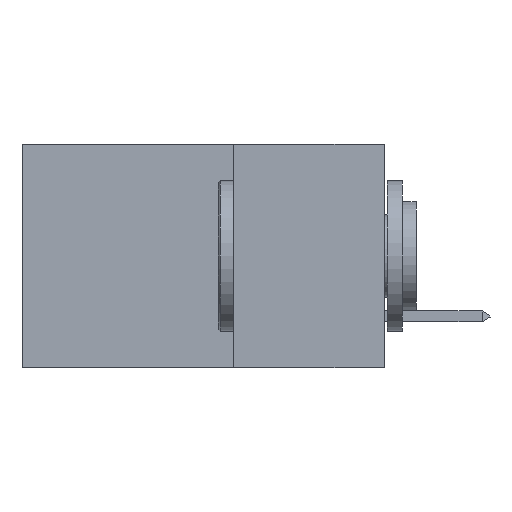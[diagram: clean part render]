
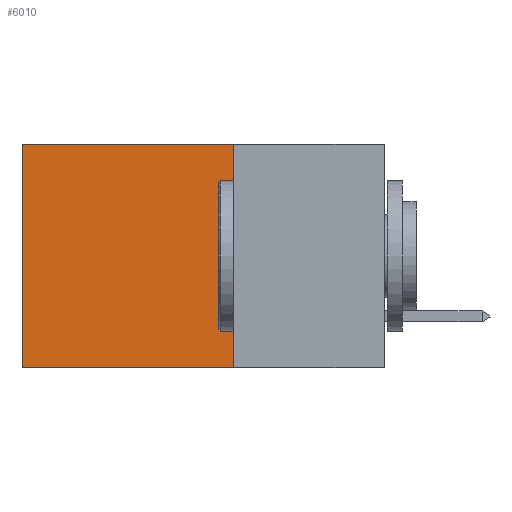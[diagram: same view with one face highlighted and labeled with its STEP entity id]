
A CAD part, left-side view. The second image highlights one B-rep face of the part: STEP entity #6010.
In plain terms, the highlighted planar face has unit normal (-1, 0, 0).
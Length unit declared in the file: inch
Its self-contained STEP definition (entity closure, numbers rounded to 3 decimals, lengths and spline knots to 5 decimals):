
#478 = EDGE_CURVE ( 'NONE', #10858, #31970, #16293, .T. ) ;
#938 = FACE_OUTER_BOUND ( 'NONE', #32908, .T. ) ;
#1613 = ORIENTED_EDGE ( 'NONE', *, *, #37143, .F. ) ;
#2845 = CARTESIAN_POINT ( 'NONE',  ( 0.2875, 0.25, 0. ) ) ;
#3653 = ORIENTED_EDGE ( 'NONE', *, *, #35912, .T. ) ;
#5150 = CARTESIAN_POINT ( 'NONE',  ( 0.2875, 0.25, -0.37 ) ) ;
#5535 = VECTOR ( 'NONE', #23234, 39.37008 ) ;
#6010 = ADVANCED_FACE ( 'NONE', ( #938 ), #42489, .F. ) ;
#9059 = VERTEX_POINT ( 'NONE', #5150 ) ;
#10151 = ORIENTED_EDGE ( 'NONE', *, *, #478, .T. ) ;
#10637 = DIRECTION ( 'NONE',  ( 0., 0., -1. ) ) ;
#10659 = EDGE_CURVE ( 'NONE', #9059, #31970, #43596, .T. ) ;
#10858 = VERTEX_POINT ( 'NONE', #28593 ) ;
#11340 = LINE ( 'NONE', #2845, #5535 ) ;
#11803 = DIRECTION ( 'NONE',  ( 0., 0., -1. ) ) ;
#12122 = DIRECTION ( 'NONE',  ( 1., 0., 0. ) ) ;
#15012 = VECTOR ( 'NONE', #10637, 39.37008 ) ;
#16293 = LINE ( 'NONE', #20194, #17301 ) ;
#17301 = VECTOR ( 'NONE', #37370, 39.37008 ) ;
#17610 = CARTESIAN_POINT ( 'NONE',  ( 0.2875, 0.25, 0. ) ) ;
#19105 = VERTEX_POINT ( 'NONE', #31724 ) ;
#20157 = AXIS2_PLACEMENT_3D ( 'NONE', #39227, #12122, #11803 ) ;
#20194 = CARTESIAN_POINT ( 'NONE',  ( 0.2875, 0.6, 0. ) ) ;
#21203 = CARTESIAN_POINT ( 'NONE',  ( 0.2875, 0.6, -0.37 ) ) ;
#23234 = DIRECTION ( 'NONE',  ( 0., 1., 0. ) ) ;
#28593 = CARTESIAN_POINT ( 'NONE',  ( 0.2875, 0.6, 0. ) ) ;
#31724 = CARTESIAN_POINT ( 'NONE',  ( 0.2875, 0.25, 0. ) ) ;
#31970 = VERTEX_POINT ( 'NONE', #21203 ) ;
#32908 = EDGE_LOOP ( 'NONE', ( #10151, #36681, #1613, #3653 ) ) ;
#33162 = LINE ( 'NONE', #17610, #15012 ) ;
#34017 = CARTESIAN_POINT ( 'NONE',  ( 0.2875, 0.25, -0.37 ) ) ;
#35912 = EDGE_CURVE ( 'NONE', #19105, #10858, #11340, .T. ) ;
#36681 = ORIENTED_EDGE ( 'NONE', *, *, #10659, .F. ) ;
#36973 = DIRECTION ( 'NONE',  ( 0., 1., 0. ) ) ;
#37143 = EDGE_CURVE ( 'NONE', #19105, #9059, #33162, .T. ) ;
#37370 = DIRECTION ( 'NONE',  ( 0., 0., -1. ) ) ;
#39227 = CARTESIAN_POINT ( 'NONE',  ( 0.2875, 0.25, 0. ) ) ;
#42489 = PLANE ( 'NONE',  #20157 ) ;
#42501 = VECTOR ( 'NONE', #36973, 39.37008 ) ;
#43596 = LINE ( 'NONE', #34017, #42501 ) ;
